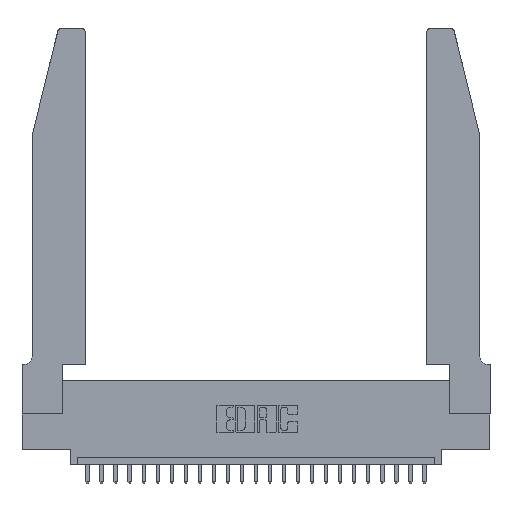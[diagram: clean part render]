
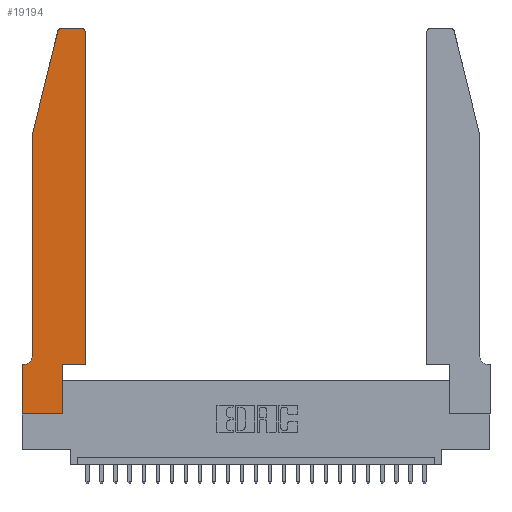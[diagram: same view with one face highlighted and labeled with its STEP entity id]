
A CAD part, top view. The second image highlights one B-rep face of the part: STEP entity #19194.
In plain terms, the highlighted planar face has unit normal (0, 0, 1).
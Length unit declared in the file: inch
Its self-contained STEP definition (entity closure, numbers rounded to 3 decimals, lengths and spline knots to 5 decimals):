
#65 = ORIENTED_EDGE ( 'NONE', *, *, #1299, .T. ) ;
#403 = AXIS2_PLACEMENT_3D ( 'NONE', #21314, #23598, #19484 ) ;
#519 = DIRECTION ( 'NONE',  ( 0., 1., 0. ) ) ;
#836 = VERTEX_POINT ( 'NONE', #10923 ) ;
#849 = ORIENTED_EDGE ( 'NONE', *, *, #18449, .T. ) ;
#1299 = EDGE_CURVE ( 'NONE', #6238, #21210, #16587, .T. ) ;
#1390 = CARTESIAN_POINT ( 'NONE',  ( 0.0055, 0.35, 0.37 ) ) ;
#1543 = CARTESIAN_POINT ( 'NONE',  ( 0.4205, 2.72, 0.37 ) ) ;
#1738 = VECTOR ( 'NONE', #12061, 39.37008 ) ;
#2348 = CARTESIAN_POINT ( 'NONE',  ( 0., 0.35, 0.37 ) ) ;
#2425 = CARTESIAN_POINT ( 'NONE',  ( 0.4505, 0.35, 0.37 ) ) ;
#2553 = CARTESIAN_POINT ( 'NONE',  ( 0.25487, 2.72718, 0.37 ) ) ;
#2733 = DIRECTION ( 'NONE',  ( -1., 0., 0. ) ) ;
#2769 = LINE ( 'NONE', #19704, #18096 ) ;
#3029 = LINE ( 'NONE', #11392, #22438 ) ;
#3980 = VECTOR ( 'NONE', #519, 39.37008 ) ;
#4237 = EDGE_CURVE ( 'NONE', #24941, #4728, #23288, .T. ) ;
#4333 = DIRECTION ( 'NONE',  ( 1., 0., 0. ) ) ;
#4388 = VERTEX_POINT ( 'NONE', #2425 ) ;
#4728 = VERTEX_POINT ( 'NONE', #11229 ) ;
#4881 = VECTOR ( 'NONE', #13705, 39.37008 ) ;
#4926 = CARTESIAN_POINT ( 'NONE',  ( 0.0755, 0.42, 0.37 ) ) ;
#5218 = ORIENTED_EDGE ( 'NONE', *, *, #18187, .T. ) ;
#5906 = DIRECTION ( 'NONE',  ( 0., 0., 1. ) ) ;
#6062 = VERTEX_POINT ( 'NONE', #11812 ) ;
#6238 = VERTEX_POINT ( 'NONE', #11945 ) ;
#6432 = LINE ( 'NONE', #15534, #1738 ) ;
#6674 = ORIENTED_EDGE ( 'NONE', *, *, #4237, .T. ) ;
#7472 = ORIENTED_EDGE ( 'NONE', *, *, #19153, .T. ) ;
#7731 = CARTESIAN_POINT ( 'NONE',  ( 0.4505, 0.35, 0.37 ) ) ;
#7852 = DIRECTION ( 'NONE',  ( -1., 0., 0. ) ) ;
#8082 = EDGE_LOOP ( 'NONE', ( #17152, #65, #5218, #14553, #18235, #849, #20656, #6674, #21033, #23324, #7472, #17933 ) ) ;
#8701 = DIRECTION ( 'NONE',  ( 0., -1., 0. ) ) ;
#9338 = AXIS2_PLACEMENT_3D ( 'NONE', #1543, #5906, #19938 ) ;
#9704 = CARTESIAN_POINT ( 'NONE',  ( 0., 0., 0.37 ) ) ;
#9712 = CARTESIAN_POINT ( 'NONE',  ( 0.0755, 2., 0.37 ) ) ;
#10582 = CARTESIAN_POINT ( 'NONE',  ( 0., 0.35, 0.37 ) ) ;
#10665 = DIRECTION ( 'NONE',  ( 0., 0., 1. ) ) ;
#10923 = CARTESIAN_POINT ( 'NONE',  ( 0.4205, 2.75, 0.37 ) ) ;
#11229 = CARTESIAN_POINT ( 'NONE',  ( 0.2865, 0., 0.37 ) ) ;
#11392 = CARTESIAN_POINT ( 'NONE',  ( 0.2605, 2.75, 0.37 ) ) ;
#11812 = CARTESIAN_POINT ( 'NONE',  ( 0.4505, 2.72, 0.37 ) ) ;
#11945 = CARTESIAN_POINT ( 'NONE',  ( 0.284, 2.75, 0.37 ) ) ;
#12061 = DIRECTION ( 'NONE',  ( 1., 0., 0. ) ) ;
#12257 = EDGE_CURVE ( 'NONE', #4728, #21506, #12783, .T. ) ;
#12684 = VECTOR ( 'NONE', #8701, 39.37008 ) ;
#12783 = LINE ( 'NONE', #24020, #3980 ) ;
#12840 = EDGE_CURVE ( 'NONE', #6062, #836, #20875, .T. ) ;
#12985 = VECTOR ( 'NONE', #21911, 39.37008 ) ;
#13399 = AXIS2_PLACEMENT_3D ( 'NONE', #20033, #22127, #7852 ) ;
#13705 = DIRECTION ( 'NONE',  ( -0.239, -0.971, 0. ) ) ;
#14057 = CARTESIAN_POINT ( 'NONE',  ( 0.2865, 0.35, 0.37 ) ) ;
#14553 = ORIENTED_EDGE ( 'NONE', *, *, #19340, .T. ) ;
#14992 = VERTEX_POINT ( 'NONE', #4926 ) ;
#15534 = CARTESIAN_POINT ( 'NONE',  ( 0.4505, 0.35, 0.37 ) ) ;
#15674 = DIRECTION ( 'NONE',  ( 0., -1., 0. ) ) ;
#16089 = LINE ( 'NONE', #16568, #12684 ) ;
#16167 = LINE ( 'NONE', #9712, #4881 ) ;
#16568 = CARTESIAN_POINT ( 'NONE',  ( 0.0755, 2., 0.37 ) ) ;
#16587 = CIRCLE ( 'NONE', #403, 0.03 ) ;
#17152 = ORIENTED_EDGE ( 'NONE', *, *, #23142, .T. ) ;
#17660 = VECTOR ( 'NONE', #19584, 39.37008 ) ;
#17668 = FACE_OUTER_BOUND ( 'NONE', #8082, .T. ) ;
#17933 = ORIENTED_EDGE ( 'NONE', *, *, #12840, .T. ) ;
#17956 = EDGE_CURVE ( 'NONE', #21506, #4388, #6432, .T. ) ;
#18096 = VECTOR ( 'NONE', #15674, 39.37008 ) ;
#18187 = EDGE_CURVE ( 'NONE', #21210, #22289, #16167, .T. ) ;
#18235 = ORIENTED_EDGE ( 'NONE', *, *, #23406, .T. ) ;
#18449 = EDGE_CURVE ( 'NONE', #24301, #21766, #25250, .T. ) ;
#18668 = VECTOR ( 'NONE', #20229, 39.37008 ) ;
#18694 = PLANE ( 'NONE',  #22067 ) ;
#19153 = EDGE_CURVE ( 'NONE', #4388, #6062, #21727, .T. ) ;
#19194 = ADVANCED_FACE ( 'NONE', ( #17668 ), #18694, .T. ) ;
#19340 = EDGE_CURVE ( 'NONE', #22289, #14992, #16089, .T. ) ;
#19484 = DIRECTION ( 'NONE',  ( 1., 0., 0. ) ) ;
#19584 = DIRECTION ( 'NONE',  ( 1., 0., 0. ) ) ;
#19704 = CARTESIAN_POINT ( 'NONE',  ( 0., 0., 0.37 ) ) ;
#19938 = DIRECTION ( 'NONE',  ( 1., 0., 0. ) ) ;
#20033 = CARTESIAN_POINT ( 'NONE',  ( 0.0055, 0.42, 0.37 ) ) ;
#20128 = CARTESIAN_POINT ( 'NONE',  ( 0.0755, 0.35, 0.37 ) ) ;
#20229 = DIRECTION ( 'NONE',  ( -1., 0., 0. ) ) ;
#20349 = CARTESIAN_POINT ( 'NONE',  ( 0.0755, 2., 0.37 ) ) ;
#20656 = ORIENTED_EDGE ( 'NONE', *, *, #22666, .T. ) ;
#20875 = CIRCLE ( 'NONE', #9338, 0.03 ) ;
#21033 = ORIENTED_EDGE ( 'NONE', *, *, #12257, .T. ) ;
#21210 = VERTEX_POINT ( 'NONE', #2553 ) ;
#21314 = CARTESIAN_POINT ( 'NONE',  ( 0.284, 2.72, 0.37 ) ) ;
#21506 = VERTEX_POINT ( 'NONE', #14057 ) ;
#21727 = LINE ( 'NONE', #7731, #12985 ) ;
#21766 = VERTEX_POINT ( 'NONE', #2348 ) ;
#21911 = DIRECTION ( 'NONE',  ( 0., 1., 0. ) ) ;
#22067 = AXIS2_PLACEMENT_3D ( 'NONE', #10582, #10665, #4333 ) ;
#22127 = DIRECTION ( 'NONE',  ( 0., 0., -1. ) ) ;
#22289 = VERTEX_POINT ( 'NONE', #20349 ) ;
#22438 = VECTOR ( 'NONE', #2733, 39.37008 ) ;
#22650 = CARTESIAN_POINT ( 'NONE',  ( 0., 0., 0.37 ) ) ;
#22666 = EDGE_CURVE ( 'NONE', #21766, #24941, #2769, .T. ) ;
#23142 = EDGE_CURVE ( 'NONE', #836, #6238, #3029, .T. ) ;
#23288 = LINE ( 'NONE', #9704, #17660 ) ;
#23324 = ORIENTED_EDGE ( 'NONE', *, *, #17956, .T. ) ;
#23406 = EDGE_CURVE ( 'NONE', #14992, #24301, #24952, .T. ) ;
#23598 = DIRECTION ( 'NONE',  ( 0., 0., 1. ) ) ;
#24020 = CARTESIAN_POINT ( 'NONE',  ( 0.2865, 0.35, 0.37 ) ) ;
#24301 = VERTEX_POINT ( 'NONE', #1390 ) ;
#24941 = VERTEX_POINT ( 'NONE', #22650 ) ;
#24952 = CIRCLE ( 'NONE', #13399, 0.07 ) ;
#25250 = LINE ( 'NONE', #20128, #18668 ) ;
